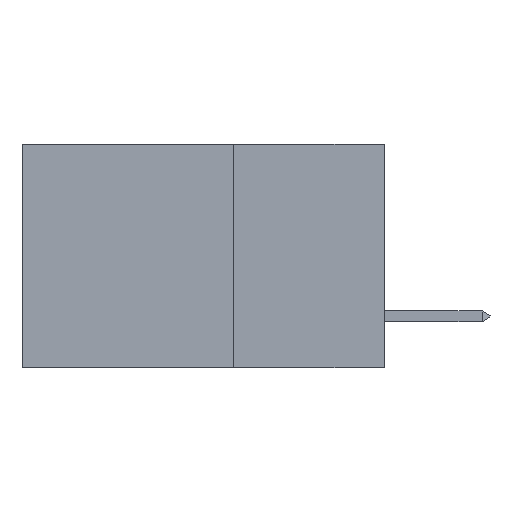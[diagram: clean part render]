
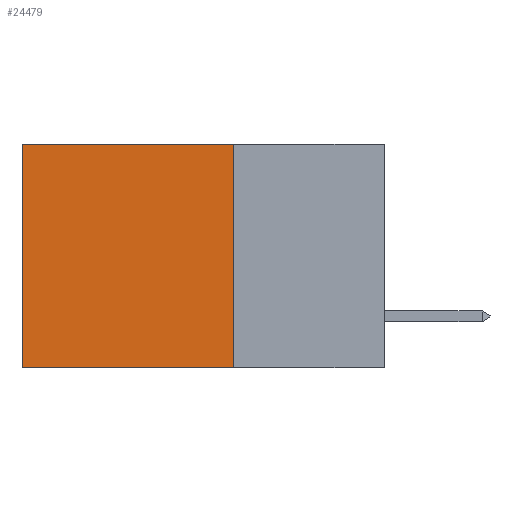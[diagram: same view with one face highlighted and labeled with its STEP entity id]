
A CAD part, left-side view. The second image highlights one B-rep face of the part: STEP entity #24479.
In plain terms, the highlighted planar face has unit normal (-1, 0, 0).
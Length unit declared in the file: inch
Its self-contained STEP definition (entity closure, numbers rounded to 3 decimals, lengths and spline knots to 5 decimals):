
#2049 = VERTEX_POINT ( 'NONE', #7633 ) ;
#2323 = EDGE_CURVE ( 'NONE', #35629, #9068, #7188, .T. ) ;
#3342 = DIRECTION ( 'NONE',  ( 0., 0., -1. ) ) ;
#3356 = LINE ( 'NONE', #34387, #34584 ) ;
#4821 = EDGE_CURVE ( 'NONE', #2049, #23176, #24377, .T. ) ;
#7188 = LINE ( 'NONE', #34611, #37080 ) ;
#7633 = CARTESIAN_POINT ( 'NONE',  ( 0.2875, 0.25, 0. ) ) ;
#8153 = CARTESIAN_POINT ( 'NONE',  ( 0.2875, 0.25, -0.37 ) ) ;
#8190 = PLANE ( 'NONE',  #15821 ) ;
#9068 = VERTEX_POINT ( 'NONE', #36518 ) ;
#11194 = FACE_OUTER_BOUND ( 'NONE', #13971, .T. ) ;
#12323 = EDGE_CURVE ( 'NONE', #2049, #35629, #27965, .T. ) ;
#12762 = CARTESIAN_POINT ( 'NONE',  ( 0.2875, 0.25, 0. ) ) ;
#13971 = EDGE_LOOP ( 'NONE', ( #37474, #19304, #33688, #34043 ) ) ;
#14389 = DIRECTION ( 'NONE',  ( 1., 0., 0. ) ) ;
#15821 = AXIS2_PLACEMENT_3D ( 'NONE', #32597, #14389, #26603 ) ;
#16188 = EDGE_CURVE ( 'NONE', #23176, #9068, #3356, .T. ) ;
#17441 = CARTESIAN_POINT ( 'NONE',  ( 0.2875, 0.6, 0. ) ) ;
#19304 = ORIENTED_EDGE ( 'NONE', *, *, #2323, .F. ) ;
#22212 = DIRECTION ( 'NONE',  ( 0., 1., 0. ) ) ;
#23176 = VERTEX_POINT ( 'NONE', #17441 ) ;
#24377 = LINE ( 'NONE', #39396, #33586 ) ;
#24479 = ADVANCED_FACE ( 'NONE', ( #11194 ), #8190, .F. ) ;
#26603 = DIRECTION ( 'NONE',  ( 0., 0., -1. ) ) ;
#27965 = LINE ( 'NONE', #12762, #36707 ) ;
#31374 = DIRECTION ( 'NONE',  ( 0., 0., -1. ) ) ;
#32597 = CARTESIAN_POINT ( 'NONE',  ( 0.2875, 0.25, 0. ) ) ;
#33586 = VECTOR ( 'NONE', #33978, 39.37008 ) ;
#33688 = ORIENTED_EDGE ( 'NONE', *, *, #12323, .F. ) ;
#33978 = DIRECTION ( 'NONE',  ( 0., 1., 0. ) ) ;
#34043 = ORIENTED_EDGE ( 'NONE', *, *, #4821, .T. ) ;
#34387 = CARTESIAN_POINT ( 'NONE',  ( 0.2875, 0.6, 0. ) ) ;
#34584 = VECTOR ( 'NONE', #31374, 39.37008 ) ;
#34611 = CARTESIAN_POINT ( 'NONE',  ( 0.2875, 0.25, -0.37 ) ) ;
#35629 = VERTEX_POINT ( 'NONE', #8153 ) ;
#36518 = CARTESIAN_POINT ( 'NONE',  ( 0.2875, 0.6, -0.37 ) ) ;
#36707 = VECTOR ( 'NONE', #3342, 39.37008 ) ;
#37080 = VECTOR ( 'NONE', #22212, 39.37008 ) ;
#37474 = ORIENTED_EDGE ( 'NONE', *, *, #16188, .T. ) ;
#39396 = CARTESIAN_POINT ( 'NONE',  ( 0.2875, 0.25, 0. ) ) ;
